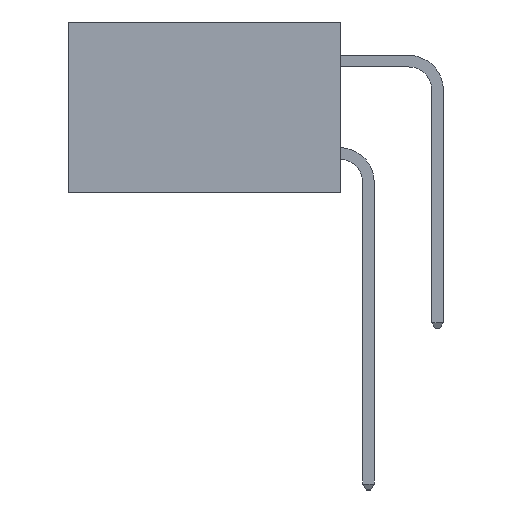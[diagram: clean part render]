
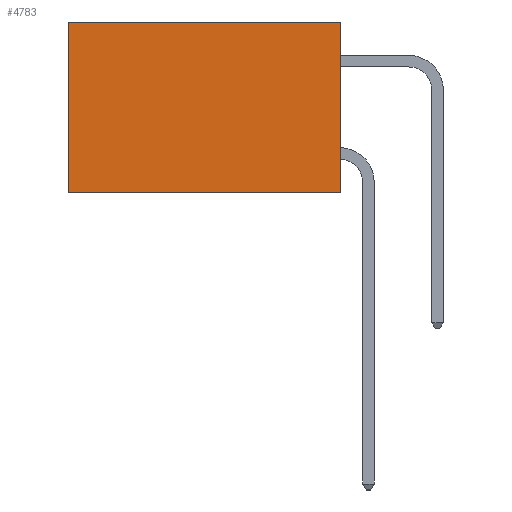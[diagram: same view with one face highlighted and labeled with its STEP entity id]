
A CAD part, left-side view. The second image highlights one B-rep face of the part: STEP entity #4783.
In plain terms, the highlighted planar face has unit normal (-1, 0, 0).
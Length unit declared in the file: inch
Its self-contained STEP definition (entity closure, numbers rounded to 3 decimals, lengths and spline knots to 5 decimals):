
#88 = CARTESIAN_POINT ( 'NONE',  ( 0.277, 0., -0.37 ) ) ;
#143 = DIRECTION ( 'NONE',  ( 0., 0., -1. ) ) ;
#641 = CARTESIAN_POINT ( 'NONE',  ( 0.277, 0.59, -0.37 ) ) ;
#694 = ORIENTED_EDGE ( 'NONE', *, *, #26303, .F. ) ;
#1202 = LINE ( 'NONE', #7060, #13320 ) ;
#2103 = FACE_OUTER_BOUND ( 'NONE', #13660, .T. ) ;
#4783 = ADVANCED_FACE ( 'NONE', ( #2103 ), #27391, .F. ) ;
#5012 = ORIENTED_EDGE ( 'NONE', *, *, #18398, .T. ) ;
#5391 = CARTESIAN_POINT ( 'NONE',  ( 0.277, 0., 0. ) ) ;
#5940 = VECTOR ( 'NONE', #7134, 39.37008 ) ;
#5950 = LINE ( 'NONE', #5391, #29377 ) ;
#7060 = CARTESIAN_POINT ( 'NONE',  ( 0.277, 0.59, -0.37 ) ) ;
#7134 = DIRECTION ( 'NONE',  ( 0., 1., 0. ) ) ;
#7362 = LINE ( 'NONE', #25482, #8077 ) ;
#7484 = EDGE_CURVE ( 'NONE', #24455, #22755, #1202, .T. ) ;
#8077 = VECTOR ( 'NONE', #27754, 39.37008 ) ;
#9306 = CARTESIAN_POINT ( 'NONE',  ( 0.277, 0., -0.37 ) ) ;
#10320 = ORIENTED_EDGE ( 'NONE', *, *, #7484, .T. ) ;
#11949 = LINE ( 'NONE', #9306, #5940 ) ;
#12084 = EDGE_CURVE ( 'NONE', #19760, #13264, #7362, .T. ) ;
#13264 = VERTEX_POINT ( 'NONE', #88 ) ;
#13320 = VECTOR ( 'NONE', #143, 39.37008 ) ;
#13660 = EDGE_LOOP ( 'NONE', ( #10320, #694, #14655, #5012 ) ) ;
#14655 = ORIENTED_EDGE ( 'NONE', *, *, #12084, .F. ) ;
#18398 = EDGE_CURVE ( 'NONE', #19760, #24455, #5950, .T. ) ;
#19418 = AXIS2_PLACEMENT_3D ( 'NONE', #27388, #27358, #27331 ) ;
#19760 = VERTEX_POINT ( 'NONE', #27534 ) ;
#22755 = VERTEX_POINT ( 'NONE', #641 ) ;
#23571 = DIRECTION ( 'NONE',  ( 0., 1., 0. ) ) ;
#24455 = VERTEX_POINT ( 'NONE', #26566 ) ;
#25482 = CARTESIAN_POINT ( 'NONE',  ( 0.277, 0., -0.37 ) ) ;
#26303 = EDGE_CURVE ( 'NONE', #13264, #22755, #11949, .T. ) ;
#26566 = CARTESIAN_POINT ( 'NONE',  ( 0.277, 0.59, 0. ) ) ;
#27331 = DIRECTION ( 'NONE',  ( 0., 0., -1. ) ) ;
#27358 = DIRECTION ( 'NONE',  ( 1., 0., 0. ) ) ;
#27388 = CARTESIAN_POINT ( 'NONE',  ( 0.277, 0., -0.37 ) ) ;
#27391 = PLANE ( 'NONE',  #19418 ) ;
#27534 = CARTESIAN_POINT ( 'NONE',  ( 0.277, 0., 0. ) ) ;
#27754 = DIRECTION ( 'NONE',  ( 0., 0., -1. ) ) ;
#29377 = VECTOR ( 'NONE', #23571, 39.37008 ) ;
